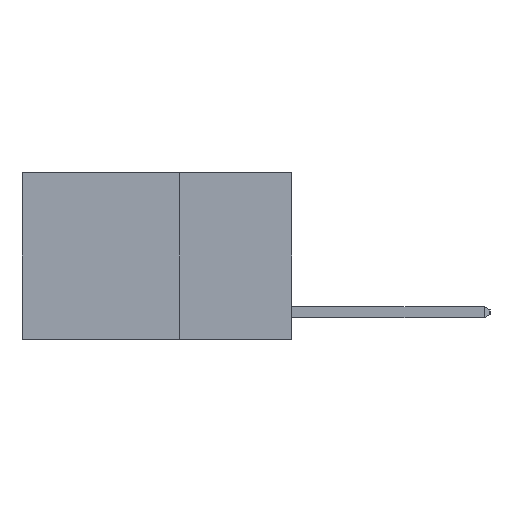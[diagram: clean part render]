
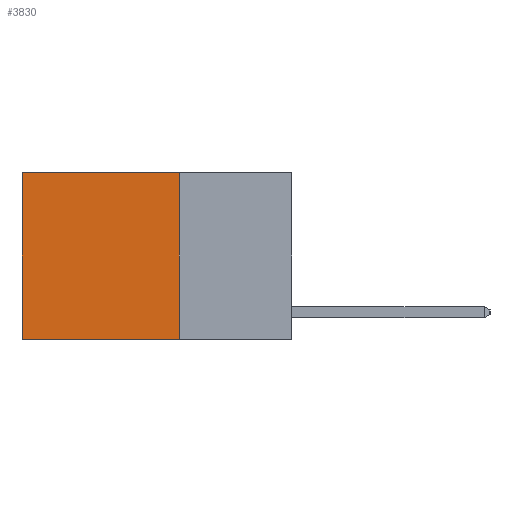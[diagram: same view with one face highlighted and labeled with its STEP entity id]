
A CAD part, left-side view. The second image highlights one B-rep face of the part: STEP entity #3830.
In plain terms, the highlighted planar face has unit normal (-1, 0, 0).
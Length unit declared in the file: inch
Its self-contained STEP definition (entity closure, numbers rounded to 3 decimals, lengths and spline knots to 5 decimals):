
#739 = EDGE_CURVE ( 'NONE', #14156, #11776, #7762, .T. ) ;
#905 = LINE ( 'NONE', #4672, #4601 ) ;
#1450 = DIRECTION ( 'NONE',  ( 0., 1., 0. ) ) ;
#1648 = VERTEX_POINT ( 'NONE', #4549 ) ;
#1697 = VECTOR ( 'NONE', #1450, 39.37008 ) ;
#2640 = FACE_OUTER_BOUND ( 'NONE', #10823, .T. ) ;
#3556 = EDGE_CURVE ( 'NONE', #6170, #14156, #13822, .T. ) ;
#3830 = ADVANCED_FACE ( 'NONE', ( #2640 ), #11485, .F. ) ;
#4546 = CARTESIAN_POINT ( 'NONE',  ( 0.2625, 0.6, -0.37 ) ) ;
#4549 = CARTESIAN_POINT ( 'NONE',  ( 0.2625, 0.6, 0. ) ) ;
#4601 = VECTOR ( 'NONE', #11644, 39.37008 ) ;
#4672 = CARTESIAN_POINT ( 'NONE',  ( 0.2625, 0.6, 0. ) ) ;
#5658 = CARTESIAN_POINT ( 'NONE',  ( 0.2625, 0.25, 0. ) ) ;
#5984 = ORIENTED_EDGE ( 'NONE', *, *, #739, .F. ) ;
#6170 = VERTEX_POINT ( 'NONE', #10623 ) ;
#6663 = ORIENTED_EDGE ( 'NONE', *, *, #9294, .T. ) ;
#6893 = DIRECTION ( 'NONE',  ( 1., 0., 0. ) ) ;
#7762 = LINE ( 'NONE', #8309, #1697 ) ;
#8309 = CARTESIAN_POINT ( 'NONE',  ( 0.2625, 0.25, -0.37 ) ) ;
#9137 = CARTESIAN_POINT ( 'NONE',  ( 0.2625, 0.25, -0.37 ) ) ;
#9294 = EDGE_CURVE ( 'NONE', #1648, #11776, #905, .T. ) ;
#9852 = CARTESIAN_POINT ( 'NONE',  ( 0.2625, 0.25, 0. ) ) ;
#10031 = VECTOR ( 'NONE', #14505, 39.37008 ) ;
#10623 = CARTESIAN_POINT ( 'NONE',  ( 0.2625, 0.25, 0. ) ) ;
#10823 = EDGE_LOOP ( 'NONE', ( #6663, #5984, #14733, #15030 ) ) ;
#11485 = PLANE ( 'NONE',  #12369 ) ;
#11644 = DIRECTION ( 'NONE',  ( 0., 0., -1. ) ) ;
#11776 = VERTEX_POINT ( 'NONE', #4546 ) ;
#12369 = AXIS2_PLACEMENT_3D ( 'NONE', #13831, #6893, #14993 ) ;
#13215 = LINE ( 'NONE', #5658, #13576 ) ;
#13576 = VECTOR ( 'NONE', #13775, 39.37008 ) ;
#13775 = DIRECTION ( 'NONE',  ( 0., 1., 0. ) ) ;
#13822 = LINE ( 'NONE', #9852, #10031 ) ;
#13831 = CARTESIAN_POINT ( 'NONE',  ( 0.2625, 0.25, 0. ) ) ;
#14156 = VERTEX_POINT ( 'NONE', #9137 ) ;
#14505 = DIRECTION ( 'NONE',  ( 0., 0., -1. ) ) ;
#14648 = EDGE_CURVE ( 'NONE', #6170, #1648, #13215, .T. ) ;
#14733 = ORIENTED_EDGE ( 'NONE', *, *, #3556, .F. ) ;
#14993 = DIRECTION ( 'NONE',  ( 0., 0., -1. ) ) ;
#15030 = ORIENTED_EDGE ( 'NONE', *, *, #14648, .T. ) ;
